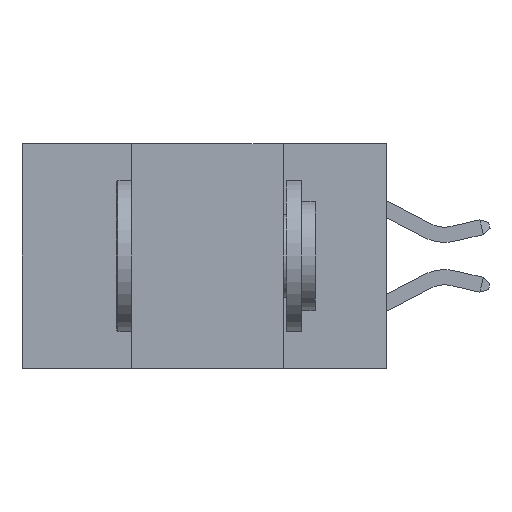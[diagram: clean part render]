
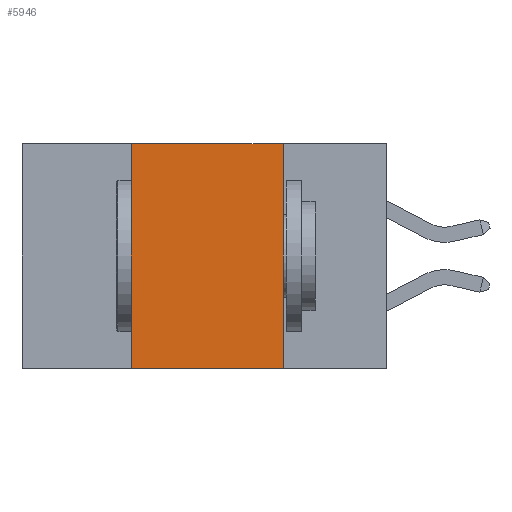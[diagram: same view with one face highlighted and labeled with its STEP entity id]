
A CAD part, left-side view. The second image highlights one B-rep face of the part: STEP entity #5946.
In plain terms, the highlighted planar face has unit normal (-1, 0, 0).
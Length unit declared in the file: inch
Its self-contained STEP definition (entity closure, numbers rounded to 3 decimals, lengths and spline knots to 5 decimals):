
#429 = VECTOR ( 'NONE', #13924, 39.37008 ) ;
#536 = EDGE_CURVE ( 'NONE', #15936, #16828, #7971, .T. ) ;
#1053 = VERTEX_POINT ( 'NONE', #14637 ) ;
#1495 = VECTOR ( 'NONE', #13255, 39.37008 ) ;
#1812 = ORIENTED_EDGE ( 'NONE', *, *, #3345, .F. ) ;
#2809 = DIRECTION ( 'NONE',  ( 0., 0., 1. ) ) ;
#3345 = EDGE_CURVE ( 'NONE', #16828, #1053, #4235, .T. ) ;
#3885 = CARTESIAN_POINT ( 'NONE',  ( 0., 0.17, 0. ) ) ;
#4235 = LINE ( 'NONE', #13724, #429 ) ;
#5596 = DIRECTION ( 'NONE',  ( 1., 0., 0. ) ) ;
#5946 = ADVANCED_FACE ( 'NONE', ( #13345 ), #6826, .F. ) ;
#6160 = CARTESIAN_POINT ( 'NONE',  ( 0., 0.6, 0. ) ) ;
#6826 = PLANE ( 'NONE',  #9496 ) ;
#6844 = VERTEX_POINT ( 'NONE', #14042 ) ;
#7636 = LINE ( 'NONE', #3885, #1495 ) ;
#7971 = LINE ( 'NONE', #9711, #14523 ) ;
#8313 = CARTESIAN_POINT ( 'NONE',  ( 0., 0.42, -0.37 ) ) ;
#8923 = CARTESIAN_POINT ( 'NONE',  ( 0., 0.42, 0. ) ) ;
#9113 = DIRECTION ( 'NONE',  ( 0., -1., 0. ) ) ;
#9496 = AXIS2_PLACEMENT_3D ( 'NONE', #6160, #5596, #15061 ) ;
#9711 = CARTESIAN_POINT ( 'NONE',  ( 0., 0.42, 0. ) ) ;
#10488 = ORIENTED_EDGE ( 'NONE', *, *, #15388, .T. ) ;
#11877 = ORIENTED_EDGE ( 'NONE', *, *, #14180, .F. ) ;
#12568 = LINE ( 'NONE', #16894, #16423 ) ;
#13255 = DIRECTION ( 'NONE',  ( 0., 0., -1. ) ) ;
#13345 = FACE_OUTER_BOUND ( 'NONE', #17135, .T. ) ;
#13724 = CARTESIAN_POINT ( 'NONE',  ( 0., 0.6, 0. ) ) ;
#13924 = DIRECTION ( 'NONE',  ( 0., -1., 0. ) ) ;
#14042 = CARTESIAN_POINT ( 'NONE',  ( 0., 0.17, -0.37 ) ) ;
#14180 = EDGE_CURVE ( 'NONE', #1053, #6844, #7636, .T. ) ;
#14523 = VECTOR ( 'NONE', #2809, 39.37008 ) ;
#14637 = CARTESIAN_POINT ( 'NONE',  ( 0., 0.17, 0. ) ) ;
#15061 = DIRECTION ( 'NONE',  ( 0., 0., -1. ) ) ;
#15388 = EDGE_CURVE ( 'NONE', #15936, #6844, #12568, .T. ) ;
#15936 = VERTEX_POINT ( 'NONE', #8313 ) ;
#16423 = VECTOR ( 'NONE', #9113, 39.37008 ) ;
#16526 = ORIENTED_EDGE ( 'NONE', *, *, #536, .F. ) ;
#16828 = VERTEX_POINT ( 'NONE', #8923 ) ;
#16894 = CARTESIAN_POINT ( 'NONE',  ( 0., 0.6, -0.37 ) ) ;
#17135 = EDGE_LOOP ( 'NONE', ( #11877, #1812, #16526, #10488 ) ) ;
